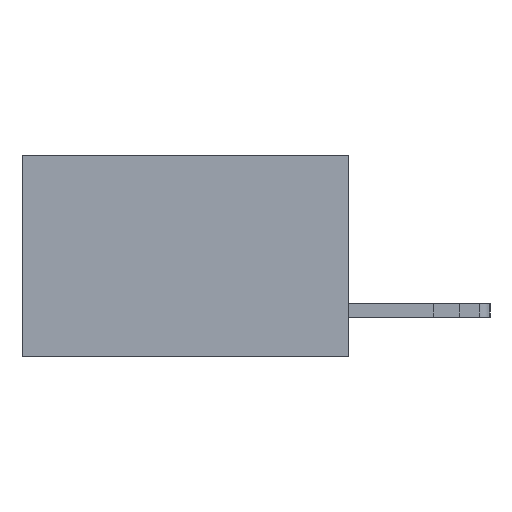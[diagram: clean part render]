
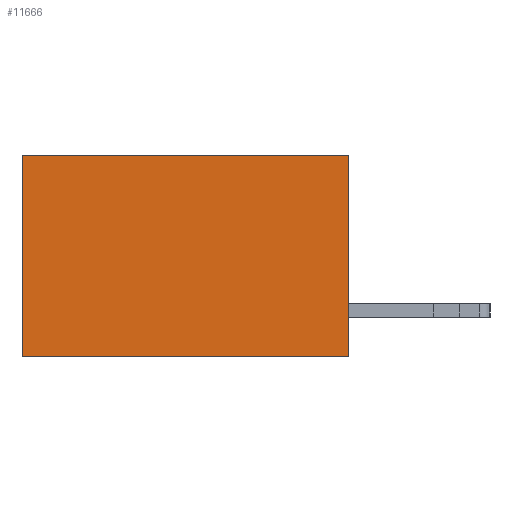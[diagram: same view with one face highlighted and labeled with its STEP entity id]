
A CAD part, left-side view. The second image highlights one B-rep face of the part: STEP entity #11666.
In plain terms, the highlighted planar face has unit normal (-1, 0, 0).
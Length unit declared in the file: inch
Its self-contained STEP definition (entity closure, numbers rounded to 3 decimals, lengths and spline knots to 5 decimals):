
#722 = EDGE_CURVE ( 'NONE', #12620, #9242, #8816, .T. ) ;
#1047 = VERTEX_POINT ( 'NONE', #5547 ) ;
#1395 = DIRECTION ( 'NONE',  ( 0., 1., 0. ) ) ;
#2349 = CARTESIAN_POINT ( 'NONE',  ( 0.298, 0., -0.37 ) ) ;
#2885 = EDGE_CURVE ( 'NONE', #1047, #12620, #15072, .T. ) ;
#3106 = ORIENTED_EDGE ( 'NONE', *, *, #722, .T. ) ;
#3479 = CARTESIAN_POINT ( 'NONE',  ( 0.298, 0., 0. ) ) ;
#3778 = CARTESIAN_POINT ( 'NONE',  ( 0.298, 0.6, 0. ) ) ;
#4472 = CARTESIAN_POINT ( 'NONE',  ( 0.298, 0., 0. ) ) ;
#5547 = CARTESIAN_POINT ( 'NONE',  ( 0.298, 0., 0. ) ) ;
#6676 = ORIENTED_EDGE ( 'NONE', *, *, #13120, .F. ) ;
#6831 = DIRECTION ( 'NONE',  ( 0., 0., -1. ) ) ;
#7439 = ORIENTED_EDGE ( 'NONE', *, *, #10982, .F. ) ;
#7771 = CARTESIAN_POINT ( 'NONE',  ( 0.298, 0., -0.37 ) ) ;
#8100 = VECTOR ( 'NONE', #6831, 39.37008 ) ;
#8816 = LINE ( 'NONE', #20551, #16832 ) ;
#9242 = VERTEX_POINT ( 'NONE', #20133 ) ;
#9447 = PLANE ( 'NONE',  #20902 ) ;
#10235 = LINE ( 'NONE', #7771, #18668 ) ;
#10263 = VECTOR ( 'NONE', #1395, 39.37008 ) ;
#10982 = EDGE_CURVE ( 'NONE', #16744, #9242, #10235, .T. ) ;
#11101 = DIRECTION ( 'NONE',  ( 0., 0., -1. ) ) ;
#11666 = ADVANCED_FACE ( 'NONE', ( #16955 ), #9447, .F. ) ;
#12433 = LINE ( 'NONE', #3479, #8100 ) ;
#12613 = DIRECTION ( 'NONE',  ( 0., 1., 0. ) ) ;
#12620 = VERTEX_POINT ( 'NONE', #3778 ) ;
#13120 = EDGE_CURVE ( 'NONE', #1047, #16744, #12433, .T. ) ;
#15072 = LINE ( 'NONE', #4472, #10263 ) ;
#16744 = VERTEX_POINT ( 'NONE', #2349 ) ;
#16832 = VECTOR ( 'NONE', #19931, 39.37008 ) ;
#16955 = FACE_OUTER_BOUND ( 'NONE', #18422, .T. ) ;
#17429 = CARTESIAN_POINT ( 'NONE',  ( 0.298, 0., 0. ) ) ;
#18422 = EDGE_LOOP ( 'NONE', ( #3106, #7439, #6676, #21006 ) ) ;
#18668 = VECTOR ( 'NONE', #12613, 39.37008 ) ;
#19931 = DIRECTION ( 'NONE',  ( 0., 0., -1. ) ) ;
#20133 = CARTESIAN_POINT ( 'NONE',  ( 0.298, 0.6, -0.37 ) ) ;
#20550 = DIRECTION ( 'NONE',  ( 1., 0., 0. ) ) ;
#20551 = CARTESIAN_POINT ( 'NONE',  ( 0.298, 0.6, 0. ) ) ;
#20902 = AXIS2_PLACEMENT_3D ( 'NONE', #17429, #20550, #11101 ) ;
#21006 = ORIENTED_EDGE ( 'NONE', *, *, #2885, .T. ) ;
